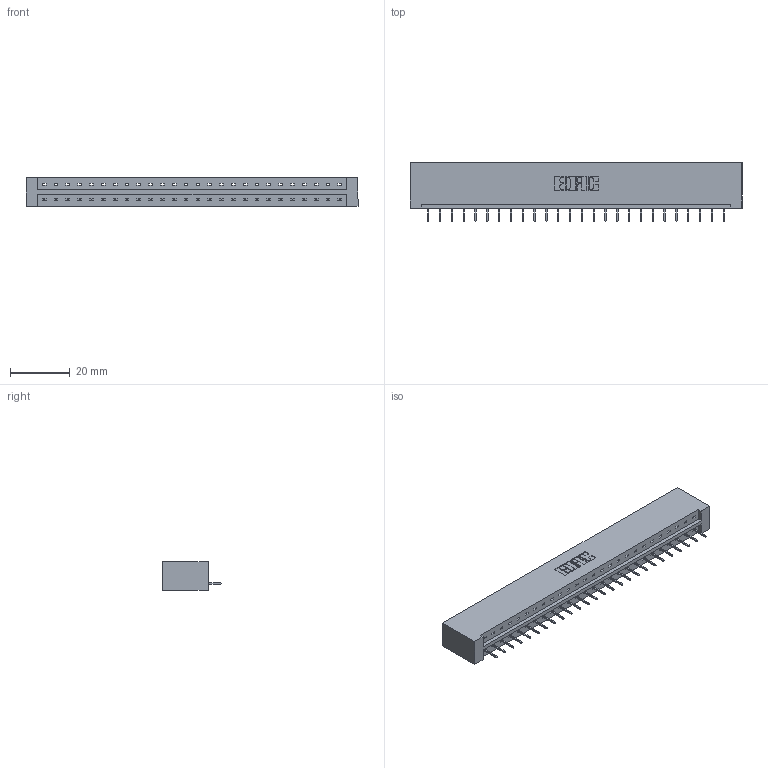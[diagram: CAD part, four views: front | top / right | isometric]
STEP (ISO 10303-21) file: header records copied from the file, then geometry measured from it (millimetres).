
FILE_DESCRIPTION (( 'STEP AP203' ), '1' );
FILE_NAME ('333-026-524-101.STEP', '2018-08-02T12:45:39', ( '' ), ( '' ), 'SwSTEP 2.0', 'SolidWorks 2016', '' );
FILE_SCHEMA (( 'CONFIG_CONTROL_DESIGN' ));
Length unit declared in the file: inch
Products named in the file (3): 333 Part_Lugless; 345-292-001_345-293-124; 333-026-524-101
Assembly tree (27 placements, depth 2):
  333-026-524-101
    333 Part_Lugless
    345-292-001_345-293-124  x26
Bounding box: 111.28 x 19.69 x 9.4 mm (x, y, z)
Volume: 11570.1 mm3; surface area: 12017.5 mm2
Topology: 27 solids, 27 shells, 1718 faces, 4967 edges, 3206 vertices
Faces by surface type: plane 1314, cylinder 404
Entity records: 17761 total; most frequent: CARTESIAN_POINT 3072, ORIENTED_EDGE 3034, DIRECTION 2617, EDGE_CURVE 1517, LINE 1401, VECTOR 1401, VERTEX_POINT 1006, AXIS2_PLACEMENT_3D 608
